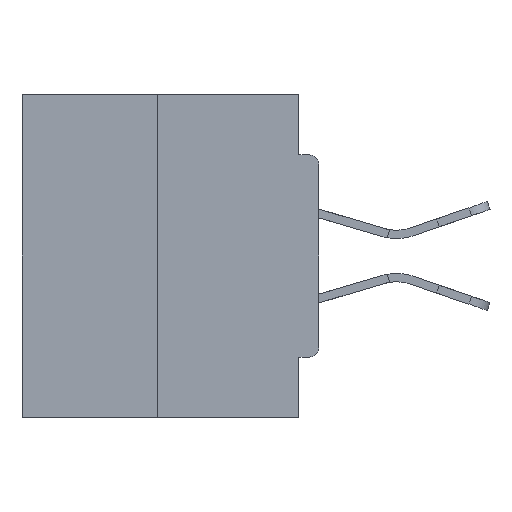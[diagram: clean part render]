
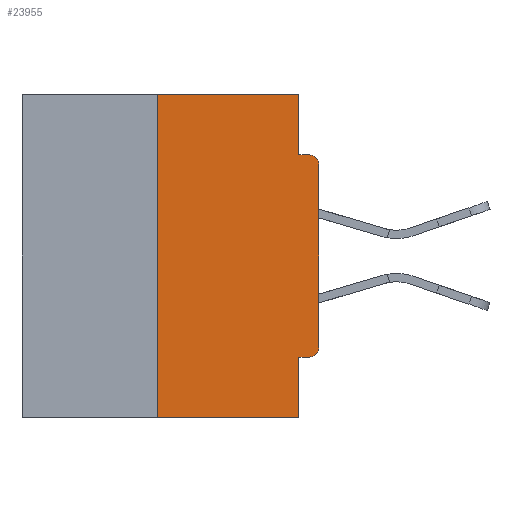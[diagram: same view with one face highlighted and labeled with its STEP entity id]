
A CAD part, left-side view. The second image highlights one B-rep face of the part: STEP entity #23955.
In plain terms, the highlighted planar face has unit normal (-1, 0, 0).
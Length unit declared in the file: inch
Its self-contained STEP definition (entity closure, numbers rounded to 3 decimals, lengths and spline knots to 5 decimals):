
#291 = EDGE_CURVE ( 'NONE', #29714, #14559, #18492, .T. ) ;
#867 = EDGE_CURVE ( 'NONE', #8599, #28053, #34075, .T. ) ;
#1263 = VECTOR ( 'NONE', #7150, 39.37008 ) ;
#1310 = CARTESIAN_POINT ( 'NONE',  ( 0., 0.46, -0.5 ) ) ;
#1904 = CARTESIAN_POINT ( 'NONE',  ( 0., 0., -0.3915 ) ) ;
#2077 = VECTOR ( 'NONE', #4139, 39.37008 ) ;
#2708 = VECTOR ( 'NONE', #8985, 39.37008 ) ;
#2900 = LINE ( 'NONE', #1310, #2708 ) ;
#3122 = AXIS2_PLACEMENT_3D ( 'NONE', #4329, #17719, #12161 ) ;
#3351 = CARTESIAN_POINT ( 'NONE',  ( 0., 0.031, -0.5 ) ) ;
#4139 = DIRECTION ( 'NONE',  ( 0., 0., 1. ) ) ;
#4329 = CARTESIAN_POINT ( 'NONE',  ( 0., 0.015, -0.3915 ) ) ;
#4908 = ORIENTED_EDGE ( 'NONE', *, *, #27906, .T. ) ;
#5062 = VERTEX_POINT ( 'NONE', #32884 ) ;
#5176 = ORIENTED_EDGE ( 'NONE', *, *, #867, .F. ) ;
#5189 = CARTESIAN_POINT ( 'NONE',  ( 0., 0.46, 0. ) ) ;
#5709 = CARTESIAN_POINT ( 'NONE',  ( 0., 0.25, 0. ) ) ;
#6631 = ORIENTED_EDGE ( 'NONE', *, *, #27033, .F. ) ;
#7150 = DIRECTION ( 'NONE',  ( 0., 0., 1. ) ) ;
#8472 = VECTOR ( 'NONE', #30605, 39.37008 ) ;
#8599 = VERTEX_POINT ( 'NONE', #16804 ) ;
#8711 = VECTOR ( 'NONE', #26443, 39.37008 ) ;
#8985 = DIRECTION ( 'NONE',  ( 0., -1., 0. ) ) ;
#9723 = CARTESIAN_POINT ( 'NONE',  ( 0., 0.015, -0.1085 ) ) ;
#9888 = EDGE_CURVE ( 'NONE', #14559, #27234, #34675, .T. ) ;
#10197 = CARTESIAN_POINT ( 'NONE',  ( 0., 0., -0.4065 ) ) ;
#10474 = EDGE_CURVE ( 'NONE', #5062, #24368, #19388, .T. ) ;
#11049 = DIRECTION ( 'NONE',  ( 1., 0., 0. ) ) ;
#11636 = FACE_OUTER_BOUND ( 'NONE', #16725, .T. ) ;
#11979 = CARTESIAN_POINT ( 'NONE',  ( 0., 0., 0. ) ) ;
#12161 = DIRECTION ( 'NONE',  ( 0., 0., -1. ) ) ;
#12418 = CARTESIAN_POINT ( 'NONE',  ( 0., 0.25, -0.5 ) ) ;
#12706 = VECTOR ( 'NONE', #16625, 39.37008 ) ;
#12742 = ORIENTED_EDGE ( 'NONE', *, *, #18462, .T. ) ;
#13036 = CARTESIAN_POINT ( 'NONE',  ( 0., 0.031, -0.5 ) ) ;
#13520 = LINE ( 'NONE', #17100, #12706 ) ;
#14317 = CARTESIAN_POINT ( 'NONE',  ( 0., 0.015, -0.0935 ) ) ;
#14559 = VERTEX_POINT ( 'NONE', #21736 ) ;
#14818 = LINE ( 'NONE', #5709, #1263 ) ;
#15142 = VERTEX_POINT ( 'NONE', #1904 ) ;
#16625 = DIRECTION ( 'NONE',  ( 0., 0., -1. ) ) ;
#16725 = EDGE_LOOP ( 'NONE', ( #33770, #6631, #18326, #19522, #19830, #21468, #12742, #4908, #5176, #27770 ) ) ;
#16804 = CARTESIAN_POINT ( 'NONE',  ( 0., 0.031, -0.0935 ) ) ;
#17100 = CARTESIAN_POINT ( 'NONE',  ( 0., 0.031, 0. ) ) ;
#17719 = DIRECTION ( 'NONE',  ( -1., 0., 0. ) ) ;
#17740 = CIRCLE ( 'NONE', #22781, 0.015 ) ;
#18206 = AXIS2_PLACEMENT_3D ( 'NONE', #24849, #11049, #27570 ) ;
#18326 = ORIENTED_EDGE ( 'NONE', *, *, #27662, .T. ) ;
#18462 = EDGE_CURVE ( 'NONE', #15142, #29142, #24853, .T. ) ;
#18492 = LINE ( 'NONE', #10197, #30732 ) ;
#19388 = LINE ( 'NONE', #5189, #32513 ) ;
#19522 = ORIENTED_EDGE ( 'NONE', *, *, #9888, .F. ) ;
#19830 = ORIENTED_EDGE ( 'NONE', *, *, #291, .F. ) ;
#20108 = DIRECTION ( 'NONE',  ( 0., 0., -1. ) ) ;
#21468 = ORIENTED_EDGE ( 'NONE', *, *, #28320, .T. ) ;
#21736 = CARTESIAN_POINT ( 'NONE',  ( 0., 0.031, -0.4065 ) ) ;
#22145 = PLANE ( 'NONE',  #18206 ) ;
#22781 = AXIS2_PLACEMENT_3D ( 'NONE', #9723, #34037, #20108 ) ;
#22911 = VERTEX_POINT ( 'NONE', #12418 ) ;
#23194 = CARTESIAN_POINT ( 'NONE',  ( 0., 0.015, -0.4065 ) ) ;
#23955 = ADVANCED_FACE ( 'NONE', ( #11636 ), #22145, .F. ) ;
#24227 = DIRECTION ( 'NONE',  ( 0., 1., 0. ) ) ;
#24368 = VERTEX_POINT ( 'NONE', #30834 ) ;
#24849 = CARTESIAN_POINT ( 'NONE',  ( 0., 0.46, 0. ) ) ;
#24853 = LINE ( 'NONE', #11979, #2077 ) ;
#26443 = DIRECTION ( 'NONE',  ( 0., -1., 0. ) ) ;
#26763 = DIRECTION ( 'NONE',  ( 0., -1., 0. ) ) ;
#27033 = EDGE_CURVE ( 'NONE', #22911, #5062, #14818, .T. ) ;
#27234 = VERTEX_POINT ( 'NONE', #13036 ) ;
#27570 = DIRECTION ( 'NONE',  ( 0., 0., -1. ) ) ;
#27662 = EDGE_CURVE ( 'NONE', #22911, #27234, #2900, .T. ) ;
#27770 = ORIENTED_EDGE ( 'NONE', *, *, #29510, .F. ) ;
#27906 = EDGE_CURVE ( 'NONE', #29142, #28053, #17740, .T. ) ;
#28053 = VERTEX_POINT ( 'NONE', #14317 ) ;
#28320 = EDGE_CURVE ( 'NONE', #29714, #15142, #29915, .T. ) ;
#29142 = VERTEX_POINT ( 'NONE', #33982 ) ;
#29414 = CARTESIAN_POINT ( 'NONE',  ( 0., 0., -0.0935 ) ) ;
#29510 = EDGE_CURVE ( 'NONE', #24368, #8599, #13520, .T. ) ;
#29714 = VERTEX_POINT ( 'NONE', #23194 ) ;
#29915 = CIRCLE ( 'NONE', #3122, 0.015 ) ;
#30605 = DIRECTION ( 'NONE',  ( 0., 0., -1. ) ) ;
#30732 = VECTOR ( 'NONE', #24227, 39.37008 ) ;
#30834 = CARTESIAN_POINT ( 'NONE',  ( 0., 0.031, 0. ) ) ;
#32513 = VECTOR ( 'NONE', #26763, 39.37008 ) ;
#32884 = CARTESIAN_POINT ( 'NONE',  ( 0., 0.25, 0. ) ) ;
#33770 = ORIENTED_EDGE ( 'NONE', *, *, #10474, .F. ) ;
#33982 = CARTESIAN_POINT ( 'NONE',  ( 0., 0., -0.1085 ) ) ;
#34037 = DIRECTION ( 'NONE',  ( -1., 0., 0. ) ) ;
#34075 = LINE ( 'NONE', #29414, #8711 ) ;
#34675 = LINE ( 'NONE', #3351, #8472 ) ;
